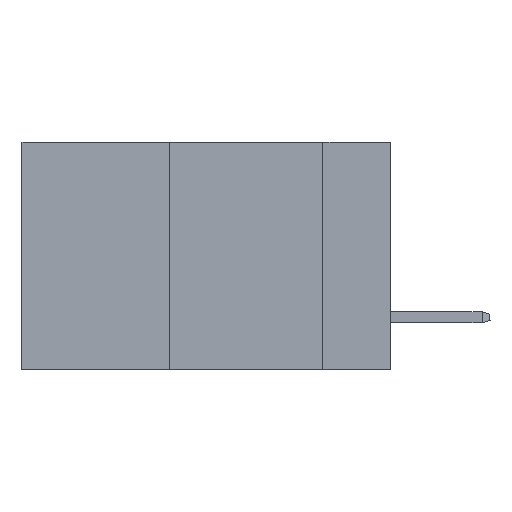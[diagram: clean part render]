
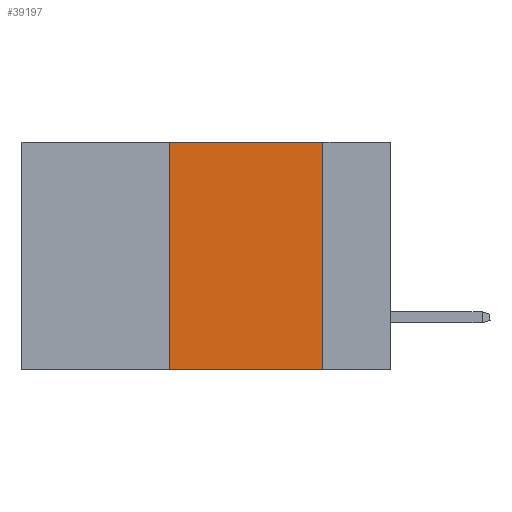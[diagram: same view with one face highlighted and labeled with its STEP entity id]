
A CAD part, left-side view. The second image highlights one B-rep face of the part: STEP entity #39197.
In plain terms, the highlighted planar face has unit normal (-1, 0, 0).
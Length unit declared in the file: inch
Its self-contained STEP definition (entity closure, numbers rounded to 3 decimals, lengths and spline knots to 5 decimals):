
#3641 = CARTESIAN_POINT ( 'NONE',  ( 0., 0.11, 0. ) ) ;
#4014 = PLANE ( 'NONE',  #19821 ) ;
#6085 = LINE ( 'NONE', #9777, #46580 ) ;
#7791 = VERTEX_POINT ( 'NONE', #3641 ) ;
#9777 = CARTESIAN_POINT ( 'NONE',  ( 0., 0.6, -0.37 ) ) ;
#10431 = VERTEX_POINT ( 'NONE', #17558 ) ;
#11887 = CARTESIAN_POINT ( 'NONE',  ( 0., 0.6, 0. ) ) ;
#12010 = ORIENTED_EDGE ( 'NONE', *, *, #16676, .F. ) ;
#13497 = DIRECTION ( 'NONE',  ( 0., -1., 0. ) ) ;
#13689 = LINE ( 'NONE', #45864, #39556 ) ;
#15546 = ORIENTED_EDGE ( 'NONE', *, *, #26418, .T. ) ;
#16447 = ORIENTED_EDGE ( 'NONE', *, *, #33834, .F. ) ;
#16676 = EDGE_CURVE ( 'NONE', #27590, #7791, #17661, .T. ) ;
#17558 = CARTESIAN_POINT ( 'NONE',  ( 0., 0.36, -0.37 ) ) ;
#17661 = LINE ( 'NONE', #18387, #42322 ) ;
#17845 = CARTESIAN_POINT ( 'NONE',  ( 0., 0.11, 0. ) ) ;
#18387 = CARTESIAN_POINT ( 'NONE',  ( 0., 0.6, 0. ) ) ;
#18395 = ORIENTED_EDGE ( 'NONE', *, *, #34039, .F. ) ;
#19663 = LINE ( 'NONE', #17845, #30790 ) ;
#19821 = AXIS2_PLACEMENT_3D ( 'NONE', #11887, #41726, #30719 ) ;
#21767 = DIRECTION ( 'NONE',  ( 0., 0., -1. ) ) ;
#24364 = EDGE_LOOP ( 'NONE', ( #16447, #12010, #18395, #15546 ) ) ;
#26418 = EDGE_CURVE ( 'NONE', #10431, #40900, #6085, .T. ) ;
#27491 = DIRECTION ( 'NONE',  ( 0., 0., 1. ) ) ;
#27590 = VERTEX_POINT ( 'NONE', #32048 ) ;
#29902 = DIRECTION ( 'NONE',  ( 0., -1., 0. ) ) ;
#30719 = DIRECTION ( 'NONE',  ( 0., 0., -1. ) ) ;
#30790 = VECTOR ( 'NONE', #21767, 39.37008 ) ;
#32048 = CARTESIAN_POINT ( 'NONE',  ( 0., 0.36, 0. ) ) ;
#32183 = CARTESIAN_POINT ( 'NONE',  ( 0., 0.11, -0.37 ) ) ;
#33834 = EDGE_CURVE ( 'NONE', #7791, #40900, #19663, .T. ) ;
#34039 = EDGE_CURVE ( 'NONE', #10431, #27590, #13689, .T. ) ;
#36531 = FACE_OUTER_BOUND ( 'NONE', #24364, .T. ) ;
#39197 = ADVANCED_FACE ( 'NONE', ( #36531 ), #4014, .F. ) ;
#39556 = VECTOR ( 'NONE', #27491, 39.37008 ) ;
#40900 = VERTEX_POINT ( 'NONE', #32183 ) ;
#41726 = DIRECTION ( 'NONE',  ( 1., 0., 0. ) ) ;
#42322 = VECTOR ( 'NONE', #29902, 39.37008 ) ;
#45864 = CARTESIAN_POINT ( 'NONE',  ( 0., 0.36, 0. ) ) ;
#46580 = VECTOR ( 'NONE', #13497, 39.37008 ) ;
